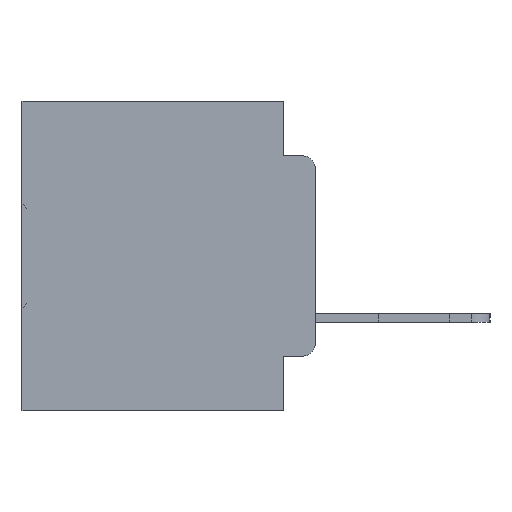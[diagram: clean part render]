
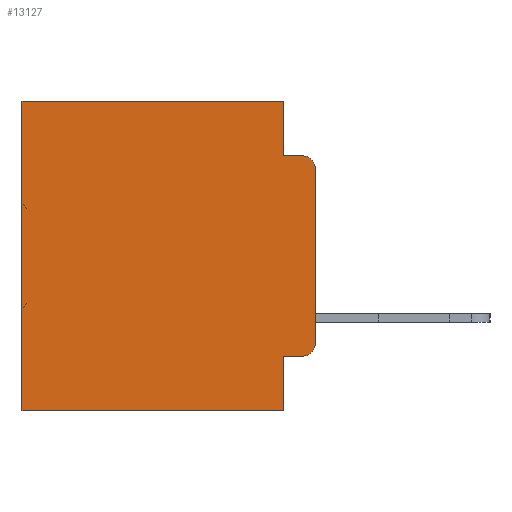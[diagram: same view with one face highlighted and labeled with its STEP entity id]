
A CAD part, left-side view. The second image highlights one B-rep face of the part: STEP entity #13127.
In plain terms, the highlighted planar face has unit normal (-1, 0, 0).
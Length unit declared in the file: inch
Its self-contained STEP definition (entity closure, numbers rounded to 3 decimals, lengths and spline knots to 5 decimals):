
#30 = VERTEX_POINT ( 'NONE', #7068 ) ;
#416 = CARTESIAN_POINT ( 'NONE',  ( 0.298, 0.473, 0. ) ) ;
#710 = DIRECTION ( 'NONE',  ( 0., -1., 0. ) ) ;
#1622 = FACE_OUTER_BOUND ( 'NONE', #9268, .T. ) ;
#1818 = CARTESIAN_POINT ( 'NONE',  ( 0.298, 0.02, -0.1085 ) ) ;
#2102 = CARTESIAN_POINT ( 'NONE',  ( 0.298, 0., -0.1085 ) ) ;
#3243 = ORIENTED_EDGE ( 'NONE', *, *, #12461, .T. ) ;
#4399 = LINE ( 'NONE', #8366, #25901 ) ;
#4613 = DIRECTION ( 'NONE',  ( 0., 0., -1. ) ) ;
#4916 = EDGE_CURVE ( 'NONE', #18918, #30, #22805, .T. ) ;
#5342 = CIRCLE ( 'NONE', #18221, 0.02 ) ;
#5505 = ORIENTED_EDGE ( 'NONE', *, *, #33705, .F. ) ;
#5706 = ORIENTED_EDGE ( 'NONE', *, *, #9603, .T. ) ;
#6303 = CARTESIAN_POINT ( 'NONE',  ( 0.298, 0., 0. ) ) ;
#6811 = EDGE_CURVE ( 'NONE', #30, #12348, #25676, .T. ) ;
#7068 = CARTESIAN_POINT ( 'NONE',  ( 0.298, 0.051, -0.0885 ) ) ;
#7122 = LINE ( 'NONE', #31065, #21226 ) ;
#7386 = ORIENTED_EDGE ( 'NONE', *, *, #35492, .T. ) ;
#8275 = CARTESIAN_POINT ( 'NONE',  ( 0.298, 0.02, -0.3915 ) ) ;
#8366 = CARTESIAN_POINT ( 'NONE',  ( 0.298, 0.051, -0.4115 ) ) ;
#9132 = DIRECTION ( 'NONE',  ( 0., 0., -1. ) ) ;
#9268 = EDGE_LOOP ( 'NONE', ( #26100, #3243, #20745, #32778, #5706, #7386, #12048, #5505, #17121, #25808 ) ) ;
#9603 = EDGE_CURVE ( 'NONE', #18918, #28944, #7122, .T. ) ;
#10107 = EDGE_CURVE ( 'NONE', #29506, #17800, #5342, .T. ) ;
#10469 = AXIS2_PLACEMENT_3D ( 'NONE', #10860, #10992, #30538 ) ;
#10780 = VECTOR ( 'NONE', #710, 39.37008 ) ;
#10860 = CARTESIAN_POINT ( 'NONE',  ( 0.298, 0., 0. ) ) ;
#10992 = DIRECTION ( 'NONE',  ( 1., 0., 0. ) ) ;
#11114 = DIRECTION ( 'NONE',  ( 0., 0., -1. ) ) ;
#12048 = ORIENTED_EDGE ( 'NONE', *, *, #16488, .F. ) ;
#12348 = VERTEX_POINT ( 'NONE', #26466 ) ;
#12461 = EDGE_CURVE ( 'NONE', #28668, #12348, #15743, .T. ) ;
#13127 = ADVANCED_FACE ( 'NONE', ( #1622 ), #22185, .F. ) ;
#14385 = DIRECTION ( 'NONE',  ( 0., 1., 0. ) ) ;
#14474 = VECTOR ( 'NONE', #24257, 39.37008 ) ;
#15743 = CIRCLE ( 'NONE', #25698, 0.02 ) ;
#16488 = EDGE_CURVE ( 'NONE', #35376, #17614, #29735, .T. ) ;
#16961 = CARTESIAN_POINT ( 'NONE',  ( 0.298, 0.473, 0. ) ) ;
#17104 = DIRECTION ( 'NONE',  ( 0., 1., 0. ) ) ;
#17121 = ORIENTED_EDGE ( 'NONE', *, *, #28196, .T. ) ;
#17614 = VERTEX_POINT ( 'NONE', #20328 ) ;
#17800 = VERTEX_POINT ( 'NONE', #34901 ) ;
#18221 = AXIS2_PLACEMENT_3D ( 'NONE', #8275, #27916, #11114 ) ;
#18918 = VERTEX_POINT ( 'NONE', #34715 ) ;
#19411 = DIRECTION ( 'NONE',  ( 0., 0., -1. ) ) ;
#19774 = DIRECTION ( 'NONE',  ( 0., 0., -1. ) ) ;
#20328 = CARTESIAN_POINT ( 'NONE',  ( 0.298, 0.473, -0.5 ) ) ;
#20745 = ORIENTED_EDGE ( 'NONE', *, *, #6811, .F. ) ;
#21226 = VECTOR ( 'NONE', #14385, 39.37008 ) ;
#21291 = LINE ( 'NONE', #6303, #35075 ) ;
#21427 = EDGE_CURVE ( 'NONE', #28668, #17800, #21291, .T. ) ;
#21492 = DIRECTION ( 'NONE',  ( -1., 0., 0. ) ) ;
#21501 = CARTESIAN_POINT ( 'NONE',  ( 0.298, 0.051, -0.4115 ) ) ;
#22185 = PLANE ( 'NONE',  #10469 ) ;
#22343 = VECTOR ( 'NONE', #17104, 39.37008 ) ;
#22398 = VECTOR ( 'NONE', #19411, 39.37008 ) ;
#22605 = CARTESIAN_POINT ( 'NONE',  ( 0.298, 0., -0.5 ) ) ;
#22805 = LINE ( 'NONE', #35184, #14474 ) ;
#24257 = DIRECTION ( 'NONE',  ( 0., 0., -1. ) ) ;
#25676 = LINE ( 'NONE', #26035, #10780 ) ;
#25698 = AXIS2_PLACEMENT_3D ( 'NONE', #1818, #21492, #4613 ) ;
#25808 = ORIENTED_EDGE ( 'NONE', *, *, #10107, .T. ) ;
#25901 = VECTOR ( 'NONE', #36081, 39.37008 ) ;
#25950 = CARTESIAN_POINT ( 'NONE',  ( 0.298, 0.02, -0.4115 ) ) ;
#26035 = CARTESIAN_POINT ( 'NONE',  ( 0.298, 0.051, -0.0885 ) ) ;
#26100 = ORIENTED_EDGE ( 'NONE', *, *, #21427, .F. ) ;
#26466 = CARTESIAN_POINT ( 'NONE',  ( 0.298, 0.02, -0.0885 ) ) ;
#26641 = VECTOR ( 'NONE', #19774, 39.37008 ) ;
#27916 = DIRECTION ( 'NONE',  ( -1., 0., 0. ) ) ;
#28196 = EDGE_CURVE ( 'NONE', #35286, #29506, #4399, .T. ) ;
#28394 = LINE ( 'NONE', #16961, #26641 ) ;
#28668 = VERTEX_POINT ( 'NONE', #2102 ) ;
#28944 = VERTEX_POINT ( 'NONE', #416 ) ;
#29506 = VERTEX_POINT ( 'NONE', #25950 ) ;
#29735 = LINE ( 'NONE', #22605, #22343 ) ;
#29791 = LINE ( 'NONE', #35891, #22398 ) ;
#30538 = DIRECTION ( 'NONE',  ( 0., 0., -1. ) ) ;
#31065 = CARTESIAN_POINT ( 'NONE',  ( 0.298, 0., 0. ) ) ;
#32778 = ORIENTED_EDGE ( 'NONE', *, *, #4916, .F. ) ;
#33090 = CARTESIAN_POINT ( 'NONE',  ( 0.298, 0.051, -0.5 ) ) ;
#33705 = EDGE_CURVE ( 'NONE', #35286, #35376, #29791, .T. ) ;
#34715 = CARTESIAN_POINT ( 'NONE',  ( 0.298, 0.051, 0. ) ) ;
#34901 = CARTESIAN_POINT ( 'NONE',  ( 0.298, 0., -0.3915 ) ) ;
#35075 = VECTOR ( 'NONE', #9132, 39.37008 ) ;
#35184 = CARTESIAN_POINT ( 'NONE',  ( 0.298, 0.051, 0. ) ) ;
#35286 = VERTEX_POINT ( 'NONE', #21501 ) ;
#35376 = VERTEX_POINT ( 'NONE', #33090 ) ;
#35492 = EDGE_CURVE ( 'NONE', #28944, #17614, #28394, .T. ) ;
#35891 = CARTESIAN_POINT ( 'NONE',  ( 0.298, 0.051, 0. ) ) ;
#36081 = DIRECTION ( 'NONE',  ( 0., -1., 0. ) ) ;
